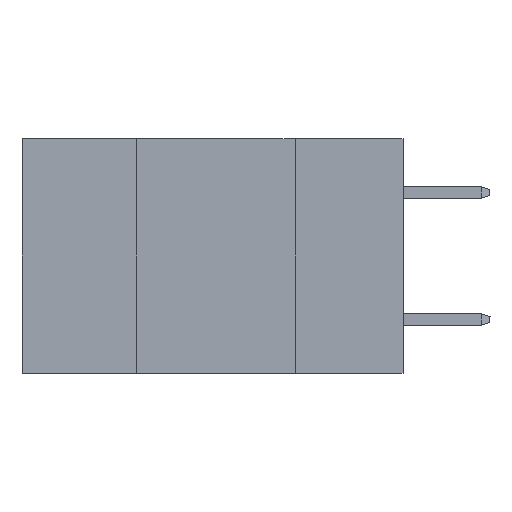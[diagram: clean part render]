
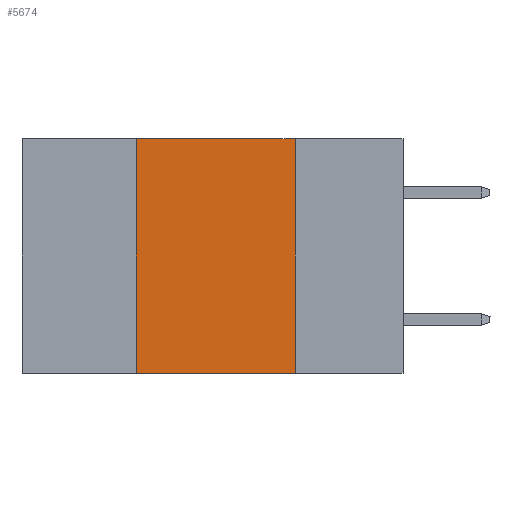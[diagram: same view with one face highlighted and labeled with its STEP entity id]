
A CAD part, left-side view. The second image highlights one B-rep face of the part: STEP entity #5674.
In plain terms, the highlighted planar face has unit normal (-1, 0, 0).
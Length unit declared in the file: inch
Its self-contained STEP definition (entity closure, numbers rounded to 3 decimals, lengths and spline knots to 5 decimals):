
#841 = VERTEX_POINT ( 'NONE', #9696 ) ;
#991 = VERTEX_POINT ( 'NONE', #3066 ) ;
#1037 = ORIENTED_EDGE ( 'NONE', *, *, #2034, .T. ) ;
#1193 = EDGE_CURVE ( 'NONE', #10500, #11785, #9199, .T. ) ;
#1451 = AXIS2_PLACEMENT_3D ( 'NONE', #4848, #16953, #15177 ) ;
#1737 = DIRECTION ( 'NONE',  ( 0., 0., -1. ) ) ;
#2034 = EDGE_CURVE ( 'NONE', #841, #991, #18201, .T. ) ;
#2418 = EDGE_CURVE ( 'NONE', #11785, #991, #6244, .T. ) ;
#3066 = CARTESIAN_POINT ( 'NONE',  ( 0., 0.17, -0.37 ) ) ;
#3140 = CARTESIAN_POINT ( 'NONE',  ( 0., 0.6, -0.37 ) ) ;
#4848 = CARTESIAN_POINT ( 'NONE',  ( 0., 0.6, 0. ) ) ;
#5024 = CARTESIAN_POINT ( 'NONE',  ( 0., 0.6, 0. ) ) ;
#5674 = ADVANCED_FACE ( 'NONE', ( #8365 ), #12159, .F. ) ;
#5972 = VECTOR ( 'NONE', #8025, 39.37008 ) ;
#6244 = LINE ( 'NONE', #9242, #12911 ) ;
#6857 = EDGE_CURVE ( 'NONE', #841, #10500, #9221, .T. ) ;
#7008 = ORIENTED_EDGE ( 'NONE', *, *, #2418, .F. ) ;
#7570 = VECTOR ( 'NONE', #7802, 39.37008 ) ;
#7802 = DIRECTION ( 'NONE',  ( 0., -1., 0. ) ) ;
#8025 = DIRECTION ( 'NONE',  ( 0., 0., 1. ) ) ;
#8365 = FACE_OUTER_BOUND ( 'NONE', #10823, .T. ) ;
#8885 = CARTESIAN_POINT ( 'NONE',  ( 0., 0.17, 0. ) ) ;
#9199 = LINE ( 'NONE', #5024, #7570 ) ;
#9221 = LINE ( 'NONE', #10674, #5972 ) ;
#9242 = CARTESIAN_POINT ( 'NONE',  ( 0., 0.17, 0. ) ) ;
#9696 = CARTESIAN_POINT ( 'NONE',  ( 0., 0.42, -0.37 ) ) ;
#10500 = VERTEX_POINT ( 'NONE', #11350 ) ;
#10674 = CARTESIAN_POINT ( 'NONE',  ( 0., 0.42, 0. ) ) ;
#10734 = VECTOR ( 'NONE', #16744, 39.37008 ) ;
#10823 = EDGE_LOOP ( 'NONE', ( #7008, #13316, #17972, #1037 ) ) ;
#11350 = CARTESIAN_POINT ( 'NONE',  ( 0., 0.42, 0. ) ) ;
#11785 = VERTEX_POINT ( 'NONE', #8885 ) ;
#12159 = PLANE ( 'NONE',  #1451 ) ;
#12911 = VECTOR ( 'NONE', #1737, 39.37008 ) ;
#13316 = ORIENTED_EDGE ( 'NONE', *, *, #1193, .F. ) ;
#15177 = DIRECTION ( 'NONE',  ( 0., 0., -1. ) ) ;
#16744 = DIRECTION ( 'NONE',  ( 0., -1., 0. ) ) ;
#16953 = DIRECTION ( 'NONE',  ( 1., 0., 0. ) ) ;
#17972 = ORIENTED_EDGE ( 'NONE', *, *, #6857, .F. ) ;
#18201 = LINE ( 'NONE', #3140, #10734 ) ;
